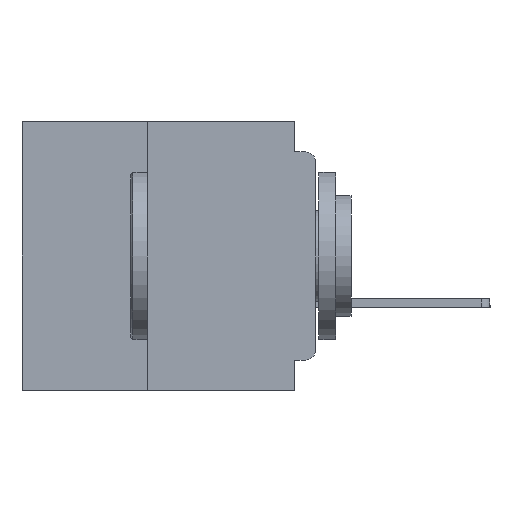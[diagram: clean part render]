
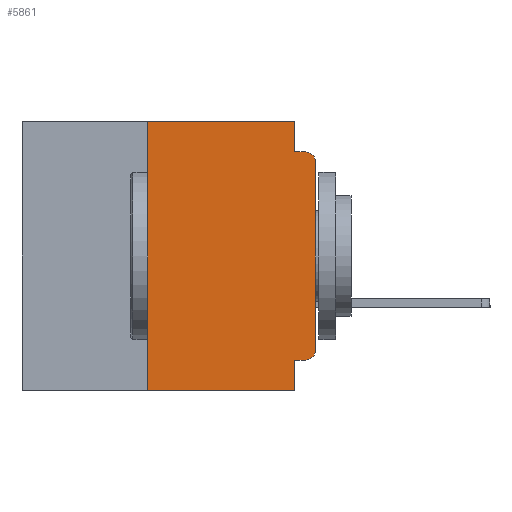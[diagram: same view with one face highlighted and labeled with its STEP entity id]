
A CAD part, left-side view. The second image highlights one B-rep face of the part: STEP entity #5861.
In plain terms, the highlighted planar face has unit normal (-1, 0, 0).
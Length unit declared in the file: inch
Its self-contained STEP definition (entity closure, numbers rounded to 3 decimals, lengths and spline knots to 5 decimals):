
#231 = EDGE_CURVE ( 'NONE', #15475, #47373, #5089, .T. ) ;
#1672 = CARTESIAN_POINT ( 'NONE',  ( 0., 0., -0.355 ) ) ;
#2528 = DIRECTION ( 'NONE',  ( 0., 0., 1. ) ) ;
#2577 = CARTESIAN_POINT ( 'NONE',  ( 0., 0.25, -0.4 ) ) ;
#2844 = CARTESIAN_POINT ( 'NONE',  ( 0., 0., -0.34 ) ) ;
#3167 = AXIS2_PLACEMENT_3D ( 'NONE', #6014, #35594, #10322 ) ;
#3765 = CARTESIAN_POINT ( 'NONE',  ( 0., 0.031, 0. ) ) ;
#4326 = ORIENTED_EDGE ( 'NONE', *, *, #231, .T. ) ;
#4969 = LINE ( 'NONE', #54410, #36055 ) ;
#5089 = CIRCLE ( 'NONE', #28867, 0.015 ) ;
#5854 = VERTEX_POINT ( 'NONE', #9865 ) ;
#5861 = ADVANCED_FACE ( 'NONE', ( #31575 ), #39395, .F. ) ;
#6014 = CARTESIAN_POINT ( 'NONE',  ( 0., 0.015, -0.34 ) ) ;
#8011 = CIRCLE ( 'NONE', #3167, 0.015 ) ;
#8361 = ORIENTED_EDGE ( 'NONE', *, *, #43041, .F. ) ;
#8851 = ORIENTED_EDGE ( 'NONE', *, *, #29551, .T. ) ;
#9397 = ORIENTED_EDGE ( 'NONE', *, *, #19823, .T. ) ;
#9865 = CARTESIAN_POINT ( 'NONE',  ( 0., 0.031, -0.355 ) ) ;
#10292 = VERTEX_POINT ( 'NONE', #3765 ) ;
#10322 = DIRECTION ( 'NONE',  ( 0., 0., -1. ) ) ;
#11395 = VECTOR ( 'NONE', #22148, 39.37008 ) ;
#11638 = VERTEX_POINT ( 'NONE', #29378 ) ;
#12264 = DIRECTION ( 'NONE',  ( 0., -1., 0. ) ) ;
#13405 = DIRECTION ( 'NONE',  ( 0., 0., -1. ) ) ;
#13902 = CARTESIAN_POINT ( 'NONE',  ( 0., 0.031, -0.045 ) ) ;
#13980 = VERTEX_POINT ( 'NONE', #16627 ) ;
#15475 = VERTEX_POINT ( 'NONE', #40508 ) ;
#16627 = CARTESIAN_POINT ( 'NONE',  ( 0., 0.031, -0.4 ) ) ;
#16762 = LINE ( 'NONE', #1672, #48988 ) ;
#17383 = CARTESIAN_POINT ( 'NONE',  ( 0., 0.437, 0. ) ) ;
#18009 = ORIENTED_EDGE ( 'NONE', *, *, #45548, .F. ) ;
#18259 = LINE ( 'NONE', #53053, #29473 ) ;
#18425 = DIRECTION ( 'NONE',  ( 1., 0., 0. ) ) ;
#18677 = ORIENTED_EDGE ( 'NONE', *, *, #46817, .F. ) ;
#18844 = ORIENTED_EDGE ( 'NONE', *, *, #39262, .F. ) ;
#19823 = EDGE_CURVE ( 'NONE', #11638, #39632, #8011, .T. ) ;
#21168 = VERTEX_POINT ( 'NONE', #2577 ) ;
#21645 = CARTESIAN_POINT ( 'NONE',  ( 0., 0.015, -0.045 ) ) ;
#22148 = DIRECTION ( 'NONE',  ( 0., 0., -1. ) ) ;
#23500 = LINE ( 'NONE', #17383, #44493 ) ;
#23526 = EDGE_CURVE ( 'NONE', #39632, #15475, #18259, .T. ) ;
#23623 = CARTESIAN_POINT ( 'NONE',  ( 0., 0.015, -0.06 ) ) ;
#23844 = EDGE_CURVE ( 'NONE', #42887, #10292, #23500, .T. ) ;
#25974 = EDGE_CURVE ( 'NONE', #10292, #26728, #44975, .T. ) ;
#26515 = DIRECTION ( 'NONE',  ( 0., -1., 0. ) ) ;
#26561 = LINE ( 'NONE', #46224, #27914 ) ;
#26728 = VERTEX_POINT ( 'NONE', #13902 ) ;
#27914 = VECTOR ( 'NONE', #50496, 39.37008 ) ;
#28867 = AXIS2_PLACEMENT_3D ( 'NONE', #23623, #39057, #13405 ) ;
#29378 = CARTESIAN_POINT ( 'NONE',  ( 0., 0.015, -0.355 ) ) ;
#29473 = VECTOR ( 'NONE', #2528, 39.37008 ) ;
#29551 = EDGE_CURVE ( 'NONE', #21168, #13980, #43974, .T. ) ;
#31575 = FACE_OUTER_BOUND ( 'NONE', #46191, .T. ) ;
#32770 = ORIENTED_EDGE ( 'NONE', *, *, #25974, .F. ) ;
#34170 = VECTOR ( 'NONE', #12264, 39.37008 ) ;
#35594 = DIRECTION ( 'NONE',  ( -1., 0., 0. ) ) ;
#36055 = VECTOR ( 'NONE', #41887, 39.37008 ) ;
#36885 = ORIENTED_EDGE ( 'NONE', *, *, #23844, .F. ) ;
#37530 = CARTESIAN_POINT ( 'NONE',  ( 0., 0.437, -0.4 ) ) ;
#38880 = CARTESIAN_POINT ( 'NONE',  ( 0., 0.031, 0. ) ) ;
#38975 = VECTOR ( 'NONE', #26515, 39.37008 ) ;
#39057 = DIRECTION ( 'NONE',  ( -1., 0., 0. ) ) ;
#39262 = EDGE_CURVE ( 'NONE', #21168, #42887, #26561, .T. ) ;
#39395 = PLANE ( 'NONE',  #43489 ) ;
#39632 = VERTEX_POINT ( 'NONE', #2844 ) ;
#40441 = ORIENTED_EDGE ( 'NONE', *, *, #23526, .T. ) ;
#40508 = CARTESIAN_POINT ( 'NONE',  ( 0., 0., -0.06 ) ) ;
#41887 = DIRECTION ( 'NONE',  ( 0., 0., -1. ) ) ;
#42887 = VERTEX_POINT ( 'NONE', #53117 ) ;
#43041 = EDGE_CURVE ( 'NONE', #5854, #13980, #4969, .T. ) ;
#43489 = AXIS2_PLACEMENT_3D ( 'NONE', #43595, #18425, #47820 ) ;
#43595 = CARTESIAN_POINT ( 'NONE',  ( 0., 0.437, 0. ) ) ;
#43974 = LINE ( 'NONE', #37530, #34170 ) ;
#44493 = VECTOR ( 'NONE', #50838, 39.37008 ) ;
#44975 = LINE ( 'NONE', #38880, #11395 ) ;
#45548 = EDGE_CURVE ( 'NONE', #11638, #5854, #16762, .T. ) ;
#46191 = EDGE_LOOP ( 'NONE', ( #40441, #4326, #18677, #32770, #36885, #18844, #8851, #8361, #18009, #9397 ) ) ;
#46224 = CARTESIAN_POINT ( 'NONE',  ( 0., 0.25, -0.4 ) ) ;
#46817 = EDGE_CURVE ( 'NONE', #26728, #47373, #50165, .T. ) ;
#47373 = VERTEX_POINT ( 'NONE', #21645 ) ;
#47820 = DIRECTION ( 'NONE',  ( 0., 0., -1. ) ) ;
#48160 = DIRECTION ( 'NONE',  ( 0., 1., 0. ) ) ;
#48988 = VECTOR ( 'NONE', #48160, 39.37008 ) ;
#50165 = LINE ( 'NONE', #51678, #38975 ) ;
#50496 = DIRECTION ( 'NONE',  ( 0., 0., 1. ) ) ;
#50838 = DIRECTION ( 'NONE',  ( 0., -1., 0. ) ) ;
#51678 = CARTESIAN_POINT ( 'NONE',  ( 0., 0., -0.045 ) ) ;
#53053 = CARTESIAN_POINT ( 'NONE',  ( 0., 0., 0. ) ) ;
#53117 = CARTESIAN_POINT ( 'NONE',  ( 0., 0.25, 0. ) ) ;
#54410 = CARTESIAN_POINT ( 'NONE',  ( 0., 0.031, -0.4 ) ) ;
